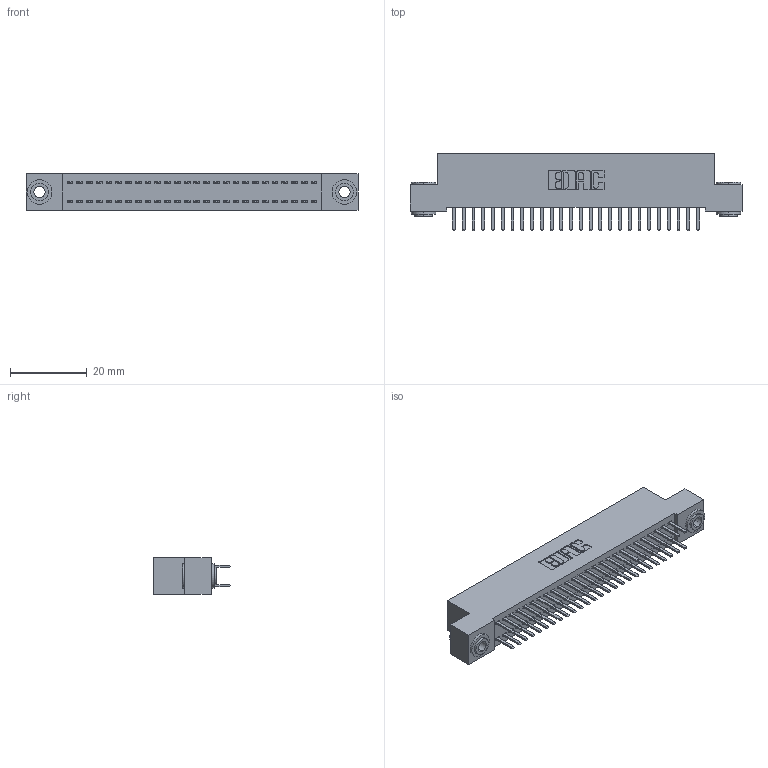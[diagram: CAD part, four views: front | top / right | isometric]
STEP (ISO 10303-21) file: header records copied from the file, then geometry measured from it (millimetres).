
FILE_DESCRIPTION (( 'STEP AP203' ), '1' );
FILE_NAME ('342-052-520-203.STEP', '2018-08-12T21:28:18', ( '' ), ( '' ), 'SwSTEP 2.0', 'SolidWorks 2016', '' );
FILE_SCHEMA (( 'CONFIG_CONTROL_DESIGN' ));
Length unit declared in the file: inch
Products named in the file (4): 342 Part_.156 TH; 345-292-001_345-293-120; 342-250-002_345-250-002-102; 342-052-520-203
Assembly tree (55 placements, depth 2):
  342-052-520-203
    342 Part_.156 TH
    345-292-001_345-293-120  x52
    342-250-002_345-250-002-102  x2
Bounding box: 86.36 x 20.02 x 9.4 mm (x, y, z)
Volume: 7683.7 mm3; surface area: 12273 mm2
Topology: 55 solids, 55 shells, 3060 faces, 8851 edges, 5758 vertices
Faces by surface type: plane 2052, cylinder 1000, cone 8
Entity records: 19428 total; most frequent: CARTESIAN_POINT 3225, ORIENTED_EDGE 3142, DIRECTION 2805, EDGE_CURVE 1571, LINE 1415, VECTOR 1415, VERTEX_POINT 1042, AXIS2_PLACEMENT_3D 695
